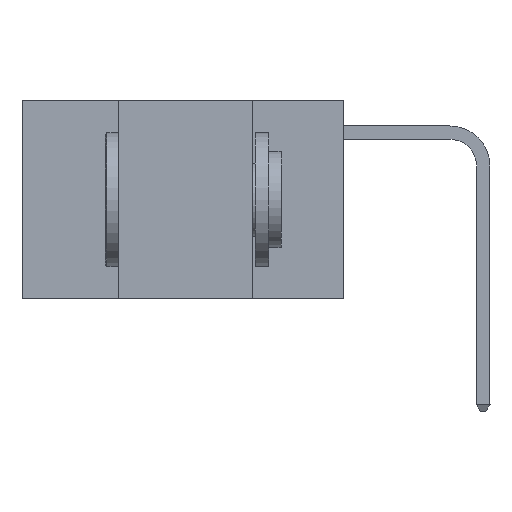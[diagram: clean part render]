
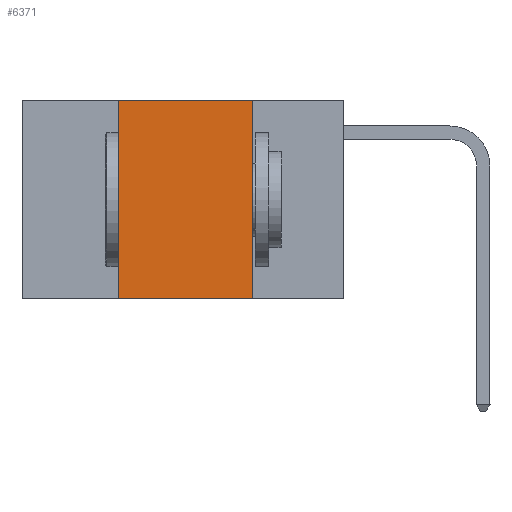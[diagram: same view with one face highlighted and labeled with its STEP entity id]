
A CAD part, left-side view. The second image highlights one B-rep face of the part: STEP entity #6371.
In plain terms, the highlighted planar face has unit normal (-1, 0, 0).
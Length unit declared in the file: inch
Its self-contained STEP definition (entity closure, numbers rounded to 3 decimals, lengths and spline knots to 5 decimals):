
#153 = VECTOR ( 'NONE', #1106, 39.37008 ) ;
#207 = CARTESIAN_POINT ( 'NONE',  ( 0., 0.42, 0. ) ) ;
#240 = VERTEX_POINT ( 'NONE', #2617 ) ;
#264 = ORIENTED_EDGE ( 'NONE', *, *, #13384, .F. ) ;
#354 = VERTEX_POINT ( 'NONE', #4994 ) ;
#1106 = DIRECTION ( 'NONE',  ( 0., 0., -1. ) ) ;
#1587 = VECTOR ( 'NONE', #3890, 39.37008 ) ;
#1799 = LINE ( 'NONE', #3958, #1587 ) ;
#2600 = CARTESIAN_POINT ( 'NONE',  ( 0., 0.6, 0. ) ) ;
#2617 = CARTESIAN_POINT ( 'NONE',  ( 0., 0.42, -0.37 ) ) ;
#2738 = VERTEX_POINT ( 'NONE', #207 ) ;
#3008 = AXIS2_PLACEMENT_3D ( 'NONE', #16141, #16041, #15725 ) ;
#3640 = LINE ( 'NONE', #3677, #153 ) ;
#3677 = CARTESIAN_POINT ( 'NONE',  ( 0., 0.17, 0. ) ) ;
#3890 = DIRECTION ( 'NONE',  ( 0., -1., 0. ) ) ;
#3958 = CARTESIAN_POINT ( 'NONE',  ( 0., 0.6, -0.37 ) ) ;
#3990 = VECTOR ( 'NONE', #15809, 39.37008 ) ;
#4994 = CARTESIAN_POINT ( 'NONE',  ( 0., 0.17, -0.37 ) ) ;
#5526 = EDGE_CURVE ( 'NONE', #240, #354, #1799, .T. ) ;
#6078 = EDGE_CURVE ( 'NONE', #240, #2738, #14133, .T. ) ;
#6371 = ADVANCED_FACE ( 'NONE', ( #9405 ), #16203, .F. ) ;
#8662 = ORIENTED_EDGE ( 'NONE', *, *, #5526, .T. ) ;
#9149 = CARTESIAN_POINT ( 'NONE',  ( 0., 0.17, 0. ) ) ;
#9405 = FACE_OUTER_BOUND ( 'NONE', #15805, .T. ) ;
#9769 = LINE ( 'NONE', #2600, #13884 ) ;
#12532 = ORIENTED_EDGE ( 'NONE', *, *, #16099, .F. ) ;
#12635 = ORIENTED_EDGE ( 'NONE', *, *, #6078, .F. ) ;
#12871 = DIRECTION ( 'NONE',  ( 0., -1., 0. ) ) ;
#13384 = EDGE_CURVE ( 'NONE', #2738, #15742, #9769, .T. ) ;
#13884 = VECTOR ( 'NONE', #12871, 39.37008 ) ;
#14133 = LINE ( 'NONE', #16284, #3990 ) ;
#15725 = DIRECTION ( 'NONE',  ( 0., 0., -1. ) ) ;
#15742 = VERTEX_POINT ( 'NONE', #9149 ) ;
#15805 = EDGE_LOOP ( 'NONE', ( #12532, #264, #12635, #8662 ) ) ;
#15809 = DIRECTION ( 'NONE',  ( 0., 0., 1. ) ) ;
#16041 = DIRECTION ( 'NONE',  ( 1., 0., 0. ) ) ;
#16099 = EDGE_CURVE ( 'NONE', #15742, #354, #3640, .T. ) ;
#16141 = CARTESIAN_POINT ( 'NONE',  ( 0., 0.6, 0. ) ) ;
#16203 = PLANE ( 'NONE',  #3008 ) ;
#16284 = CARTESIAN_POINT ( 'NONE',  ( 0., 0.42, 0. ) ) ;
